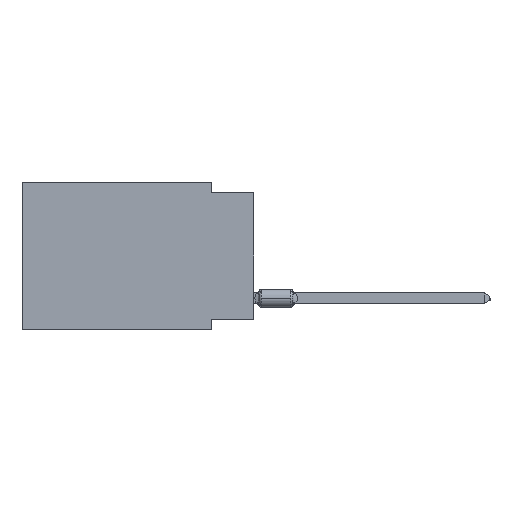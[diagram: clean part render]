
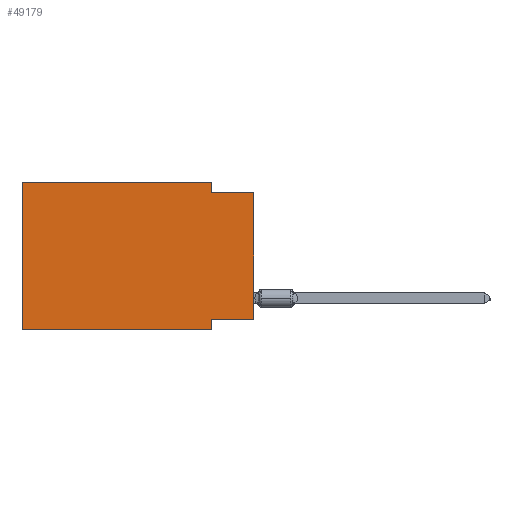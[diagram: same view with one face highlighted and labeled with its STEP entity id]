
A CAD part, left-side view. The second image highlights one B-rep face of the part: STEP entity #49179.
In plain terms, the highlighted planar face has unit normal (-1, 0, 0).
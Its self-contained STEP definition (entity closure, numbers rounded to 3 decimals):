
#645 = LINE ( 'NONE', #959, #37332 ) ;
#684 = DIRECTION ( 'NONE',  ( 0., 0., 1. ) ) ;
#848 = CARTESIAN_POINT ( 'NONE',  ( 0., 0., -0.635 ) ) ;
#959 = CARTESIAN_POINT ( 'NONE',  ( 0., 13.97, -8.89 ) ) ;
#1705 = FACE_OUTER_BOUND ( 'NONE', #3730, .T. ) ;
#2269 = EDGE_CURVE ( 'NONE', #11459, #51366, #645, .T. ) ;
#3456 = CARTESIAN_POINT ( 'NONE',  ( 0., 0., -8.255 ) ) ;
#3730 = EDGE_LOOP ( 'NONE', ( #35677, #23479, #40395, #60828, #7511, #16526, #14742, #23083 ) ) ;
#5768 = CARTESIAN_POINT ( 'NONE',  ( 0., 0., -8.255 ) ) ;
#7511 = ORIENTED_EDGE ( 'NONE', *, *, #27001, .F. ) ;
#8170 = CARTESIAN_POINT ( 'NONE',  ( 0., 2.54, -8.255 ) ) ;
#9961 = VECTOR ( 'NONE', #60516, 1000. ) ;
#11082 = LINE ( 'NONE', #46279, #58316 ) ;
#11459 = VERTEX_POINT ( 'NONE', #63558 ) ;
#11790 = PLANE ( 'NONE',  #19985 ) ;
#14742 = ORIENTED_EDGE ( 'NONE', *, *, #42487, .F. ) ;
#15312 = VERTEX_POINT ( 'NONE', #848 ) ;
#15344 = EDGE_CURVE ( 'NONE', #59034, #28502, #50399, .T. ) ;
#16526 = ORIENTED_EDGE ( 'NONE', *, *, #2269, .T. ) ;
#17646 = DIRECTION ( 'NONE',  ( 1., 0., 0. ) ) ;
#18131 = VERTEX_POINT ( 'NONE', #54833 ) ;
#18553 = LINE ( 'NONE', #28299, #56077 ) ;
#19985 = AXIS2_PLACEMENT_3D ( 'NONE', #62323, #17646, #31663 ) ;
#21223 = EDGE_CURVE ( 'NONE', #48473, #15312, #51909, .T. ) ;
#23083 = ORIENTED_EDGE ( 'NONE', *, *, #15344, .F. ) ;
#23479 = ORIENTED_EDGE ( 'NONE', *, *, #21223, .F. ) ;
#24326 = LINE ( 'NONE', #59541, #51473 ) ;
#27001 = EDGE_CURVE ( 'NONE', #11459, #18131, #54817, .T. ) ;
#28299 = CARTESIAN_POINT ( 'NONE',  ( 0., 2.54, 0. ) ) ;
#28502 = VERTEX_POINT ( 'NONE', #8170 ) ;
#29032 = CARTESIAN_POINT ( 'NONE',  ( 0., 13.97, 0. ) ) ;
#29800 = CARTESIAN_POINT ( 'NONE',  ( 0., 2.54, -0.635 ) ) ;
#31663 = DIRECTION ( 'NONE',  ( 0., 0., -1. ) ) ;
#31909 = DIRECTION ( 'NONE',  ( 0., 0., -1. ) ) ;
#33537 = VECTOR ( 'NONE', #42126, 1000. ) ;
#33608 = VECTOR ( 'NONE', #39414, 1000. ) ;
#34002 = EDGE_CURVE ( 'NONE', #55545, #48473, #18553, .T. ) ;
#35677 = ORIENTED_EDGE ( 'NONE', *, *, #46555, .T. ) ;
#37332 = VECTOR ( 'NONE', #49855, 1000. ) ;
#38233 = CARTESIAN_POINT ( 'NONE',  ( 0., 2.54, -8.89 ) ) ;
#39414 = DIRECTION ( 'NONE',  ( 0., 0., 1. ) ) ;
#40395 = ORIENTED_EDGE ( 'NONE', *, *, #34002, .F. ) ;
#42126 = DIRECTION ( 'NONE',  ( 0., -1., 0. ) ) ;
#42487 = EDGE_CURVE ( 'NONE', #28502, #51366, #11082, .T. ) ;
#43694 = LINE ( 'NONE', #53799, #33608 ) ;
#44219 = DIRECTION ( 'NONE',  ( 0., -1., 0. ) ) ;
#46279 = CARTESIAN_POINT ( 'NONE',  ( 0., 2.54, -8.89 ) ) ;
#46555 = EDGE_CURVE ( 'NONE', #59034, #15312, #43694, .T. ) ;
#47014 = CARTESIAN_POINT ( 'NONE',  ( 0., 0., -0.635 ) ) ;
#48473 = VERTEX_POINT ( 'NONE', #29800 ) ;
#49179 = ADVANCED_FACE ( 'NONE', ( #1705 ), #11790, .F. ) ;
#49855 = DIRECTION ( 'NONE',  ( 0., -1., 0. ) ) ;
#50399 = LINE ( 'NONE', #5768, #9961 ) ;
#51366 = VERTEX_POINT ( 'NONE', #38233 ) ;
#51473 = VECTOR ( 'NONE', #44219, 1000. ) ;
#51909 = LINE ( 'NONE', #47014, #33537 ) ;
#53799 = CARTESIAN_POINT ( 'NONE',  ( 0., 0., 0. ) ) ;
#54817 = LINE ( 'NONE', #29032, #56022 ) ;
#54833 = CARTESIAN_POINT ( 'NONE',  ( 0., 13.97, 0. ) ) ;
#55545 = VERTEX_POINT ( 'NONE', #63700 ) ;
#56022 = VECTOR ( 'NONE', #684, 1000. ) ;
#56077 = VECTOR ( 'NONE', #57702, 1000. ) ;
#57702 = DIRECTION ( 'NONE',  ( 0., 0., -1. ) ) ;
#58316 = VECTOR ( 'NONE', #31909, 1000. ) ;
#59034 = VERTEX_POINT ( 'NONE', #3456 ) ;
#59541 = CARTESIAN_POINT ( 'NONE',  ( 0., 13.97, 0. ) ) ;
#60516 = DIRECTION ( 'NONE',  ( 0., 1., 0. ) ) ;
#60828 = ORIENTED_EDGE ( 'NONE', *, *, #64269, .F. ) ;
#62323 = CARTESIAN_POINT ( 'NONE',  ( 0., 13.97, 0. ) ) ;
#63558 = CARTESIAN_POINT ( 'NONE',  ( 0., 13.97, -8.89 ) ) ;
#63700 = CARTESIAN_POINT ( 'NONE',  ( 0., 2.54, 0. ) ) ;
#64269 = EDGE_CURVE ( 'NONE', #18131, #55545, #24326, .T. ) ;
